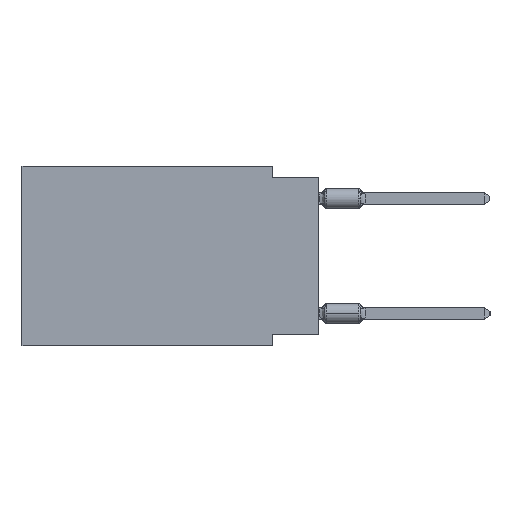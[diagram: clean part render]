
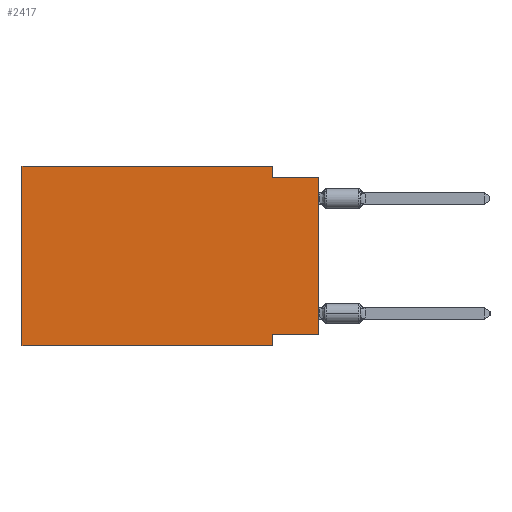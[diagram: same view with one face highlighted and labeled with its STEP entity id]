
A CAD part, left-side view. The second image highlights one B-rep face of the part: STEP entity #2417.
In plain terms, the highlighted planar face has unit normal (-1, 0, 0).
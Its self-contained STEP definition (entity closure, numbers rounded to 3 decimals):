
#1545 = EDGE_CURVE ( 'NONE', #3029, #19438, #20955, .T. ) ;
#2417 = ADVANCED_FACE ( 'NONE', ( #11928 ), #26235, .F. ) ;
#3029 = VERTEX_POINT ( 'NONE', #17327 ) ;
#3031 = VECTOR ( 'NONE', #15600, 1000. ) ;
#3332 = VERTEX_POINT ( 'NONE', #30550 ) ;
#3595 = EDGE_CURVE ( 'NONE', #19438, #19042, #32085, .T. ) ;
#3925 = CARTESIAN_POINT ( 'NONE',  ( 0., 0., -0.635 ) ) ;
#4868 = VERTEX_POINT ( 'NONE', #26945 ) ;
#5394 = CARTESIAN_POINT ( 'NONE',  ( 0., 16.383, -9.906 ) ) ;
#6206 = CARTESIAN_POINT ( 'NONE',  ( 0., 0., 0. ) ) ;
#6589 = EDGE_CURVE ( 'NONE', #3332, #4868, #19814, .T. ) ;
#7773 = CARTESIAN_POINT ( 'NONE',  ( 0., 16.383, -9.906 ) ) ;
#7987 = CARTESIAN_POINT ( 'NONE',  ( 0., 2.54, -9.906 ) ) ;
#9465 = DIRECTION ( 'NONE',  ( 0., -1., 0. ) ) ;
#9591 = EDGE_CURVE ( 'NONE', #34864, #32887, #21391, .T. ) ;
#9886 = CARTESIAN_POINT ( 'NONE',  ( 0., 2.54, 0. ) ) ;
#9977 = EDGE_CURVE ( 'NONE', #3332, #34864, #21015, .T. ) ;
#10232 = DIRECTION ( 'NONE',  ( 0., -1., 0. ) ) ;
#11022 = DIRECTION ( 'NONE',  ( 0., 0., 1. ) ) ;
#11733 = EDGE_CURVE ( 'NONE', #19042, #4868, #29128, .T. ) ;
#11928 = FACE_OUTER_BOUND ( 'NONE', #14692, .T. ) ;
#12328 = VECTOR ( 'NONE', #11022, 1000. ) ;
#13022 = ORIENTED_EDGE ( 'NONE', *, *, #27448, .T. ) ;
#13210 = ORIENTED_EDGE ( 'NONE', *, *, #9591, .F. ) ;
#13338 = CARTESIAN_POINT ( 'NONE',  ( 0., 2.54, -0.635 ) ) ;
#13402 = VECTOR ( 'NONE', #9465, 1000. ) ;
#14168 = ORIENTED_EDGE ( 'NONE', *, *, #31180, .F. ) ;
#14488 = DIRECTION ( 'NONE',  ( 0., 0., 1. ) ) ;
#14506 = VERTEX_POINT ( 'NONE', #7773 ) ;
#14622 = VECTOR ( 'NONE', #23811, 1000. ) ;
#14692 = EDGE_LOOP ( 'NONE', ( #24914, #21938, #17042, #32255, #14168, #13022, #13210, #29725 ) ) ;
#15600 = DIRECTION ( 'NONE',  ( 0., 1., 0. ) ) ;
#17042 = ORIENTED_EDGE ( 'NONE', *, *, #3595, .F. ) ;
#17327 = CARTESIAN_POINT ( 'NONE',  ( 0., 16.383, 0. ) ) ;
#18523 = DIRECTION ( 'NONE',  ( 0., 0., -1. ) ) ;
#19042 = VERTEX_POINT ( 'NONE', #13338 ) ;
#19438 = VERTEX_POINT ( 'NONE', #9886 ) ;
#19798 = AXIS2_PLACEMENT_3D ( 'NONE', #22854, #33758, #28395 ) ;
#19814 = LINE ( 'NONE', #6206, #12328 ) ;
#20955 = LINE ( 'NONE', #23291, #14622 ) ;
#21015 = LINE ( 'NONE', #29210, #3031 ) ;
#21391 = LINE ( 'NONE', #7987, #23585 ) ;
#21547 = DIRECTION ( 'NONE',  ( 0., 0., -1. ) ) ;
#21938 = ORIENTED_EDGE ( 'NONE', *, *, #11733, .F. ) ;
#22181 = VECTOR ( 'NONE', #21547, 1000. ) ;
#22753 = CARTESIAN_POINT ( 'NONE',  ( 0., 16.383, 0. ) ) ;
#22854 = CARTESIAN_POINT ( 'NONE',  ( 0., 16.383, 0. ) ) ;
#23291 = CARTESIAN_POINT ( 'NONE',  ( 0., 16.383, 0. ) ) ;
#23585 = VECTOR ( 'NONE', #18523, 1000. ) ;
#23811 = DIRECTION ( 'NONE',  ( 0., -1., 0. ) ) ;
#24384 = LINE ( 'NONE', #5394, #31639 ) ;
#24914 = ORIENTED_EDGE ( 'NONE', *, *, #6589, .T. ) ;
#25116 = CARTESIAN_POINT ( 'NONE',  ( 0., 2.54, -9.906 ) ) ;
#26235 = PLANE ( 'NONE',  #19798 ) ;
#26945 = CARTESIAN_POINT ( 'NONE',  ( 0., 0., -0.635 ) ) ;
#27448 = EDGE_CURVE ( 'NONE', #14506, #32887, #24384, .T. ) ;
#28395 = DIRECTION ( 'NONE',  ( 0., 0., -1. ) ) ;
#28877 = VECTOR ( 'NONE', #14488, 1000. ) ;
#29128 = LINE ( 'NONE', #3925, #13402 ) ;
#29210 = CARTESIAN_POINT ( 'NONE',  ( 0., 0., -9.271 ) ) ;
#29333 = CARTESIAN_POINT ( 'NONE',  ( 0., 2.54, -9.271 ) ) ;
#29725 = ORIENTED_EDGE ( 'NONE', *, *, #9977, .F. ) ;
#30550 = CARTESIAN_POINT ( 'NONE',  ( 0., 0., -9.271 ) ) ;
#30806 = LINE ( 'NONE', #22753, #28877 ) ;
#31180 = EDGE_CURVE ( 'NONE', #14506, #3029, #30806, .T. ) ;
#31639 = VECTOR ( 'NONE', #10232, 1000. ) ;
#32085 = LINE ( 'NONE', #32471, #22181 ) ;
#32255 = ORIENTED_EDGE ( 'NONE', *, *, #1545, .F. ) ;
#32471 = CARTESIAN_POINT ( 'NONE',  ( 0., 2.54, 0. ) ) ;
#32887 = VERTEX_POINT ( 'NONE', #25116 ) ;
#33758 = DIRECTION ( 'NONE',  ( 1., 0., 0. ) ) ;
#34864 = VERTEX_POINT ( 'NONE', #29333 ) ;
